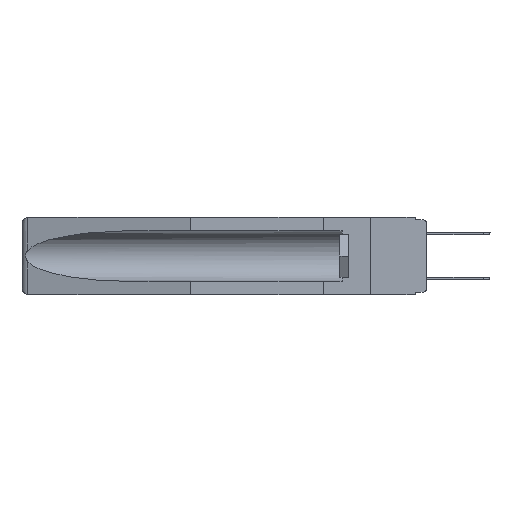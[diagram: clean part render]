
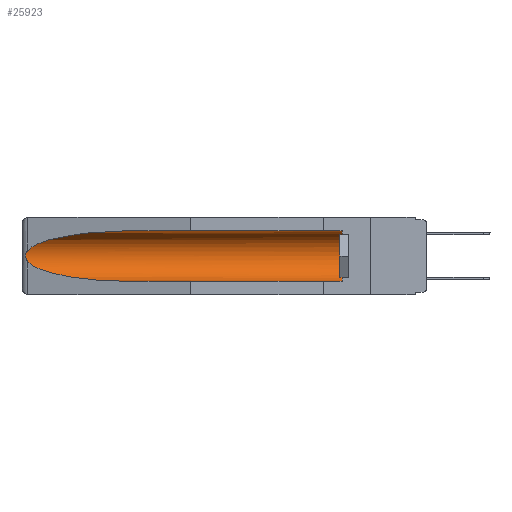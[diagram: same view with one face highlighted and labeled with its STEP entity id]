
A CAD part, left-side view. The second image highlights one B-rep face of the part: STEP entity #25923.
In plain terms, the highlighted cylindrical face has radius 2.857 mm (diameter 5.715 mm), a partial arc.
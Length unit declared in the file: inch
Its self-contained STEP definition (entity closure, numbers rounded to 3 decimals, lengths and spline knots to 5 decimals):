
#391 = EDGE_CURVE ( 'NONE', #7218, #656, #13017, .T. ) ;
#497 = DIRECTION ( 'NONE',  ( 0., 1., 0. ) ) ;
#545 = CYLINDRICAL_SURFACE ( 'NONE', #11001, 0.1125 ) ;
#656 = VERTEX_POINT ( 'NONE', #5418 ) ;
#869 = CIRCLE ( 'NONE', #11274, 0.1125 ) ;
#1587 = CARTESIAN_POINT ( 'NONE',  ( 0.26537, 1.52718, -0.14972 ) ) ;
#1777 = ORIENTED_EDGE ( 'NONE', *, *, #391, .T. ) ;
#1965 = VECTOR ( 'NONE', #497, 39.37008 ) ;
#2658 = CARTESIAN_POINT ( 'NONE',  ( 0.21114, 1.30732, -0.059 ) ) ;
#3605 = CARTESIAN_POINT ( 'NONE',  ( 0.2675, 1.53308, -0.16763 ) ) ;
#3776 = CARTESIAN_POINT ( 'NONE',  ( 0.26597, 1.52961, -0.15275 ) ) ;
#4877 = B_SPLINE_CURVE_WITH_KNOTS ( 'NONE', 3,
 ( #1587, #3776, #16296, #12119, #3605, #27041, #27128, #7870, #18465, #14254 ),
 .UNSPECIFIED., .F., .F.,
 ( 4, 2, 2, 2, 4 ),
 ( 0., 0.00029, 0.00058, 0.00087, 0.00117 ),
 .UNSPECIFIED. ) ;
#5291 = EDGE_CURVE ( 'NONE', #21123, #24767, #869, .T. ) ;
#5418 = CARTESIAN_POINT ( 'NONE',  ( 0.26537, 1.52718, -0.14972 ) ) ;
#6339 = CARTESIAN_POINT ( 'NONE',  ( 0.155, 0.126, -0.284 ) ) ;
#6921 = CARTESIAN_POINT ( 'NONE',  ( 0.26537, 1.52718, -0.14972 ) ) ;
#6997 = CARTESIAN_POINT ( 'NONE',  ( 0.155, 0.126, -0.1715 ) ) ;
#7218 = VERTEX_POINT ( 'NONE', #18111 ) ;
#7250 = DIRECTION ( 'NONE',  ( 0., 1., 0. ) ) ;
#7870 = CARTESIAN_POINT ( 'NONE',  ( 0.26655, 1.53094, -0.18657 ) ) ;
#8506 = CARTESIAN_POINT ( 'NONE',  ( 0.155, 1.07973, -0.284 ) ) ;
#8600 = CARTESIAN_POINT ( 'NONE',  ( 0.21114, 1.30732, -0.284 ) ) ;
#9148 = VERTEX_POINT ( 'NONE', #9712 ) ;
#9222 = CARTESIAN_POINT ( 'NONE',  ( 0.25451, 1.48313, -0.09465 ) ) ;
#9712 = CARTESIAN_POINT ( 'NONE',  ( 0.155, 1.07973, -0.284 ) ) ;
#10809 = CARTESIAN_POINT ( 'NONE',  ( 0.25451, 1.48313, -0.24835 ) ) ;
#11001 = AXIS2_PLACEMENT_3D ( 'NONE', #16681, #25542, #12678 ) ;
#11227 = CARTESIAN_POINT ( 'NONE',  ( 0.155, -0.30754, -0.284 ) ) ;
#11274 = AXIS2_PLACEMENT_3D ( 'NONE', #6997, #13481, #19907 ) ;
#12119 = CARTESIAN_POINT ( 'NONE',  ( 0.2673, 1.5327, -0.16383 ) ) ;
#12413 = FACE_OUTER_BOUND ( 'NONE', #24349, .T. ) ;
#12678 = DIRECTION ( 'NONE',  ( 0., 0., 1. ) ) ;
#12692 = EDGE_CURVE ( 'NONE', #656, #24066, #4877, .T. ) ;
#13017 =( BOUNDED_CURVE ( )  B_SPLINE_CURVE ( 3, ( #26066, #2658, #9222, #6921 ),
 .UNSPECIFIED., .F., .F. ) 
 B_SPLINE_CURVE_WITH_KNOTS ( ( 4, 4 ),
 ( 4.71239, 6.08839 ),
 .UNSPECIFIED. ) 
 CURVE ( )  GEOMETRIC_REPRESENTATION_ITEM ( )  RATIONAL_B_SPLINE_CURVE ( ( 1., 0.848, 0.848, 1. ) ) 
 REPRESENTATION_ITEM ( '' )  );
#13061 = EDGE_CURVE ( 'NONE', #24066, #9148, #26674, .T. ) ;
#13481 = DIRECTION ( 'NONE',  ( 0., -1., 0. ) ) ;
#13544 = LINE ( 'NONE', #11227, #1965 ) ;
#13649 = CARTESIAN_POINT ( 'NONE',  ( 0.155, -0.30754, -0.059 ) ) ;
#13982 = ORIENTED_EDGE ( 'NONE', *, *, #13061, .T. ) ;
#14254 = CARTESIAN_POINT ( 'NONE',  ( 0.26537, 1.52718, -0.19328 ) ) ;
#14266 = EDGE_CURVE ( 'NONE', #21123, #9148, #13544, .T. ) ;
#14976 = CARTESIAN_POINT ( 'NONE',  ( 0.26537, 1.52718, -0.19328 ) ) ;
#16296 = CARTESIAN_POINT ( 'NONE',  ( 0.26654, 1.53092, -0.15636 ) ) ;
#16360 = ORIENTED_EDGE ( 'NONE', *, *, #12692, .T. ) ;
#16681 = CARTESIAN_POINT ( 'NONE',  ( 0.155, -0.30754, -0.1715 ) ) ;
#17267 = CARTESIAN_POINT ( 'NONE',  ( 0.26537, 1.52718, -0.19328 ) ) ;
#18111 = CARTESIAN_POINT ( 'NONE',  ( 0.155, 1.07973, -0.059 ) ) ;
#18465 = CARTESIAN_POINT ( 'NONE',  ( 0.26597, 1.5296, -0.19026 ) ) ;
#18733 = LINE ( 'NONE', #13649, #19749 ) ;
#19749 = VECTOR ( 'NONE', #7250, 39.37008 ) ;
#19907 = DIRECTION ( 'NONE',  ( 0., 0., 1. ) ) ;
#20136 = ORIENTED_EDGE ( 'NONE', *, *, #5291, .T. ) ;
#21123 = VERTEX_POINT ( 'NONE', #6339 ) ;
#21614 = CARTESIAN_POINT ( 'NONE',  ( 0.155, 0.126, -0.059 ) ) ;
#21883 = ORIENTED_EDGE ( 'NONE', *, *, #14266, .F. ) ;
#24034 = ORIENTED_EDGE ( 'NONE', *, *, #26854, .T. ) ;
#24066 = VERTEX_POINT ( 'NONE', #17267 ) ;
#24349 = EDGE_LOOP ( 'NONE', ( #1777, #16360, #13982, #21883, #20136, #24034 ) ) ;
#24767 = VERTEX_POINT ( 'NONE', #21614 ) ;
#25542 = DIRECTION ( 'NONE',  ( 0., 1., 0. ) ) ;
#25923 = ADVANCED_FACE ( 'NONE', ( #12413 ), #545, .F. ) ;
#26066 = CARTESIAN_POINT ( 'NONE',  ( 0.155, 1.07973, -0.059 ) ) ;
#26674 =( BOUNDED_CURVE ( )  B_SPLINE_CURVE ( 3, ( #14976, #10809, #8600, #8506 ),
 .UNSPECIFIED., .F., .F. ) 
 B_SPLINE_CURVE_WITH_KNOTS ( ( 4, 4 ),
 ( 0.1948, 1.5708 ),
 .UNSPECIFIED. ) 
 CURVE ( )  GEOMETRIC_REPRESENTATION_ITEM ( )  RATIONAL_B_SPLINE_CURVE ( ( 1., 0.848, 0.848, 1. ) ) 
 REPRESENTATION_ITEM ( '' )  );
#26854 = EDGE_CURVE ( 'NONE', #24767, #7218, #18733, .T. ) ;
#27041 = CARTESIAN_POINT ( 'NONE',  ( 0.2675, 1.53308, -0.17534 ) ) ;
#27128 = CARTESIAN_POINT ( 'NONE',  ( 0.2673, 1.53269, -0.17917 ) ) ;
